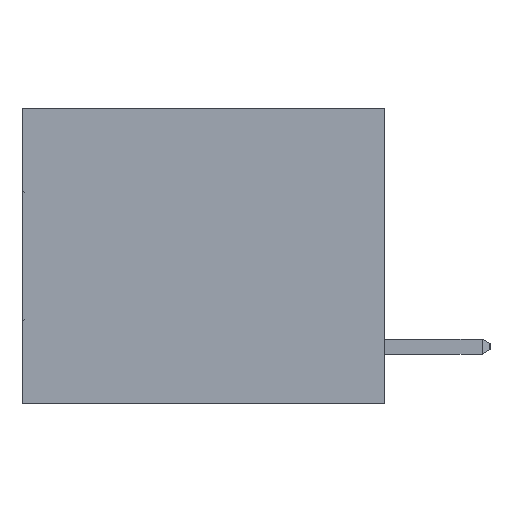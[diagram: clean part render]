
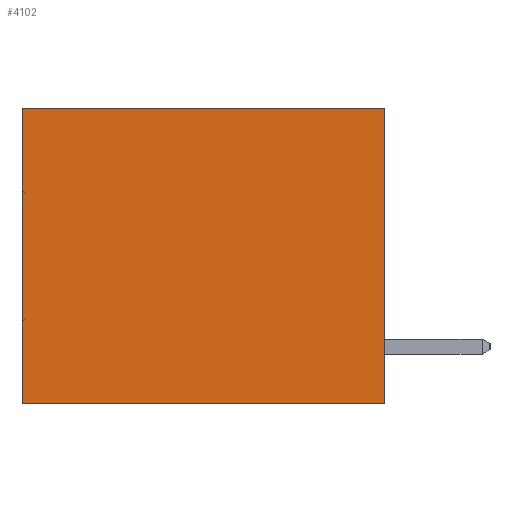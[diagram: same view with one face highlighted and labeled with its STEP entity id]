
A CAD part, left-side view. The second image highlights one B-rep face of the part: STEP entity #4102.
In plain terms, the highlighted planar face has unit normal (-1, 0, 0).
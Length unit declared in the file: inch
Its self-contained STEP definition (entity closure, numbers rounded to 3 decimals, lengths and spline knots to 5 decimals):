
#1988 = CARTESIAN_POINT ( 'NONE',  ( 0.3165, 0., 0. ) ) ;
#2034 = LINE ( 'NONE', #32814, #2861 ) ;
#2508 = ORIENTED_EDGE ( 'NONE', *, *, #28089, .F. ) ;
#2861 = VECTOR ( 'NONE', #12127, 39.37008 ) ;
#4102 = ADVANCED_FACE ( 'NONE', ( #17987 ), #12907, .F. ) ;
#4256 = EDGE_LOOP ( 'NONE', ( #18087, #32281, #2508, #23781 ) ) ;
#4913 = CARTESIAN_POINT ( 'NONE',  ( 0.3165, 0., 0. ) ) ;
#5086 = VERTEX_POINT ( 'NONE', #8701 ) ;
#6614 = EDGE_CURVE ( 'NONE', #6806, #5086, #21034, .T. ) ;
#6806 = VERTEX_POINT ( 'NONE', #28777 ) ;
#8701 = CARTESIAN_POINT ( 'NONE',  ( 0.3165, 0.6, -0.49 ) ) ;
#9038 = DIRECTION ( 'NONE',  ( 0., 0., -1. ) ) ;
#10030 = CARTESIAN_POINT ( 'NONE',  ( 0.3165, 0., -0.49 ) ) ;
#12127 = DIRECTION ( 'NONE',  ( 0., 0., -1. ) ) ;
#12182 = EDGE_CURVE ( 'NONE', #28509, #14599, #16480, .T. ) ;
#12907 = PLANE ( 'NONE',  #23993 ) ;
#14599 = VERTEX_POINT ( 'NONE', #28891 ) ;
#15404 = CARTESIAN_POINT ( 'NONE',  ( 0.3165, 0., -0.49 ) ) ;
#16091 = VECTOR ( 'NONE', #22717, 39.37008 ) ;
#16408 = CARTESIAN_POINT ( 'NONE',  ( 0.3165, 0., -0.49 ) ) ;
#16480 = LINE ( 'NONE', #1988, #16091 ) ;
#17831 = DIRECTION ( 'NONE',  ( 0., 0., -1. ) ) ;
#17987 = FACE_OUTER_BOUND ( 'NONE', #4256, .T. ) ;
#18087 = ORIENTED_EDGE ( 'NONE', *, *, #20933, .T. ) ;
#18624 = VECTOR ( 'NONE', #28330, 39.37008 ) ;
#20933 = EDGE_CURVE ( 'NONE', #14599, #5086, #2034, .T. ) ;
#21034 = LINE ( 'NONE', #10030, #18624 ) ;
#22717 = DIRECTION ( 'NONE',  ( 0., 1., 0. ) ) ;
#23781 = ORIENTED_EDGE ( 'NONE', *, *, #12182, .T. ) ;
#23993 = AXIS2_PLACEMENT_3D ( 'NONE', #15404, #31100, #17831 ) ;
#26142 = VECTOR ( 'NONE', #9038, 39.37008 ) ;
#28089 = EDGE_CURVE ( 'NONE', #28509, #6806, #29396, .T. ) ;
#28330 = DIRECTION ( 'NONE',  ( 0., 1., 0. ) ) ;
#28509 = VERTEX_POINT ( 'NONE', #4913 ) ;
#28777 = CARTESIAN_POINT ( 'NONE',  ( 0.3165, 0., -0.49 ) ) ;
#28891 = CARTESIAN_POINT ( 'NONE',  ( 0.3165, 0.6, 0. ) ) ;
#29396 = LINE ( 'NONE', #16408, #26142 ) ;
#31100 = DIRECTION ( 'NONE',  ( 1., 0., 0. ) ) ;
#32281 = ORIENTED_EDGE ( 'NONE', *, *, #6614, .F. ) ;
#32814 = CARTESIAN_POINT ( 'NONE',  ( 0.3165, 0.6, -0.49 ) ) ;
